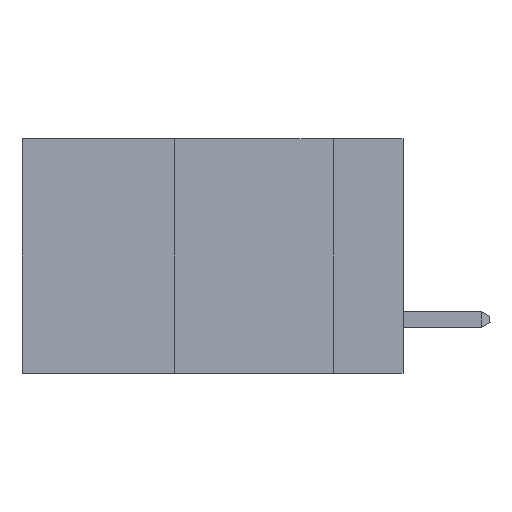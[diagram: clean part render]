
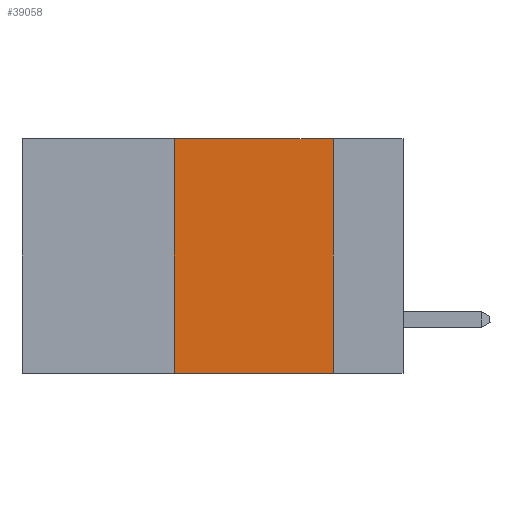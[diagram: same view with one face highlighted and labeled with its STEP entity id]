
A CAD part, left-side view. The second image highlights one B-rep face of the part: STEP entity #39058.
In plain terms, the highlighted planar face has unit normal (-1, 0, 0).
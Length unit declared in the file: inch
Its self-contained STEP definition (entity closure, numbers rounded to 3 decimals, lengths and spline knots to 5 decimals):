
#78 = VERTEX_POINT ( 'NONE', #5913 ) ;
#609 = CARTESIAN_POINT ( 'NONE',  ( 0., 0.36, 0. ) ) ;
#967 = EDGE_CURVE ( 'NONE', #33436, #78, #8697, .T. ) ;
#4093 = VECTOR ( 'NONE', #4386, 39.37008 ) ;
#4386 = DIRECTION ( 'NONE',  ( 0., 0., 1. ) ) ;
#5913 = CARTESIAN_POINT ( 'NONE',  ( 0., 0.11, -0.37 ) ) ;
#8697 = LINE ( 'NONE', #33726, #47277 ) ;
#9976 = LINE ( 'NONE', #32833, #38582 ) ;
#11073 = VECTOR ( 'NONE', #11195, 39.37008 ) ;
#11137 = DIRECTION ( 'NONE',  ( 0., 0., -1. ) ) ;
#11195 = DIRECTION ( 'NONE',  ( 0., -1., 0. ) ) ;
#14602 = LINE ( 'NONE', #609, #4093 ) ;
#15152 = ORIENTED_EDGE ( 'NONE', *, *, #21515, .F. ) ;
#16414 = ORIENTED_EDGE ( 'NONE', *, *, #967, .T. ) ;
#16825 = FACE_OUTER_BOUND ( 'NONE', #25274, .T. ) ;
#19726 = CARTESIAN_POINT ( 'NONE',  ( 0., 0.36, 0. ) ) ;
#20261 = AXIS2_PLACEMENT_3D ( 'NONE', #46997, #28336, #46491 ) ;
#21216 = VERTEX_POINT ( 'NONE', #19726 ) ;
#21316 = CARTESIAN_POINT ( 'NONE',  ( 0., 0.11, 0. ) ) ;
#21515 = EDGE_CURVE ( 'NONE', #21216, #40627, #40284, .T. ) ;
#21809 = EDGE_CURVE ( 'NONE', #33436, #21216, #14602, .T. ) ;
#25274 = EDGE_LOOP ( 'NONE', ( #33136, #15152, #44338, #16414 ) ) ;
#25295 = EDGE_CURVE ( 'NONE', #40627, #78, #9976, .T. ) ;
#28336 = DIRECTION ( 'NONE',  ( 1., 0., 0. ) ) ;
#32833 = CARTESIAN_POINT ( 'NONE',  ( 0., 0.11, 0. ) ) ;
#33136 = ORIENTED_EDGE ( 'NONE', *, *, #25295, .F. ) ;
#33436 = VERTEX_POINT ( 'NONE', #47118 ) ;
#33726 = CARTESIAN_POINT ( 'NONE',  ( 0., 0.6, -0.37 ) ) ;
#35234 = PLANE ( 'NONE',  #20261 ) ;
#38582 = VECTOR ( 'NONE', #11137, 39.37008 ) ;
#39058 = ADVANCED_FACE ( 'NONE', ( #16825 ), #35234, .F. ) ;
#40284 = LINE ( 'NONE', #41366, #11073 ) ;
#40627 = VERTEX_POINT ( 'NONE', #21316 ) ;
#41366 = CARTESIAN_POINT ( 'NONE',  ( 0., 0.6, 0. ) ) ;
#44338 = ORIENTED_EDGE ( 'NONE', *, *, #21809, .F. ) ;
#44547 = DIRECTION ( 'NONE',  ( 0., -1., 0. ) ) ;
#46491 = DIRECTION ( 'NONE',  ( 0., 0., -1. ) ) ;
#46997 = CARTESIAN_POINT ( 'NONE',  ( 0., 0.6, 0. ) ) ;
#47118 = CARTESIAN_POINT ( 'NONE',  ( 0., 0.36, -0.37 ) ) ;
#47277 = VECTOR ( 'NONE', #44547, 39.37008 ) ;
